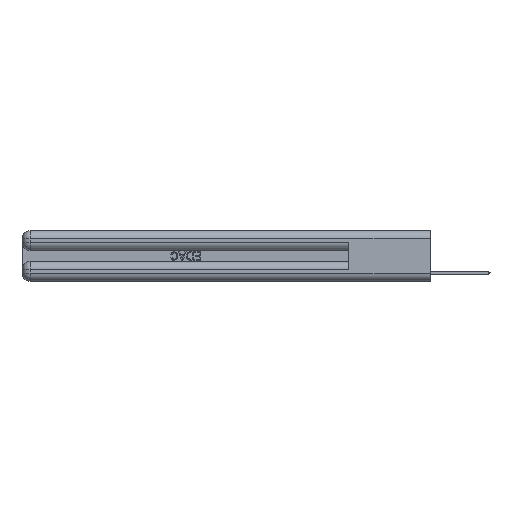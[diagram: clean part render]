
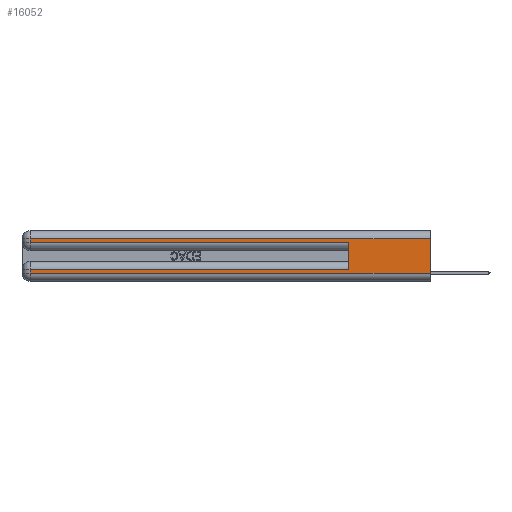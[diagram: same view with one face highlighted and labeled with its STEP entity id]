
A CAD part, left-side view. The second image highlights one B-rep face of the part: STEP entity #16052.
In plain terms, the highlighted planar face has unit normal (-1, 0, 0).
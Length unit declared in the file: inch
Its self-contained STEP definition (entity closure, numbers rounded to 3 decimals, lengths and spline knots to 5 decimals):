
#622 = VECTOR ( 'NONE', #1805, 39.37008 ) ;
#898 = VERTEX_POINT ( 'NONE', #18366 ) ;
#1225 = PLANE ( 'NONE',  #11989 ) ;
#1238 = DIRECTION ( 'NONE',  ( 0., 0., -1. ) ) ;
#1465 = DIRECTION ( 'NONE',  ( 0., 1., 0. ) ) ;
#1669 = CARTESIAN_POINT ( 'NONE',  ( 0., 2.94, 0.06 ) ) ;
#1805 = DIRECTION ( 'NONE',  ( 0., 0., -1. ) ) ;
#2607 = VECTOR ( 'NONE', #1238, 39.37008 ) ;
#2774 = CARTESIAN_POINT ( 'NONE',  ( 0., 0., 0.085 ) ) ;
#3349 = EDGE_CURVE ( 'NONE', #22937, #3726, #15953, .T. ) ;
#3726 = VERTEX_POINT ( 'NONE', #12110 ) ;
#3815 = ORIENTED_EDGE ( 'NONE', *, *, #12244, .T. ) ;
#4378 = EDGE_LOOP ( 'NONE', ( #17534, #11414, #22323, #23015, #10605, #10803, #24562, #3815 ) ) ;
#4987 = CARTESIAN_POINT ( 'NONE',  ( 0., 0., 0.285 ) ) ;
#5040 = DIRECTION ( 'NONE',  ( 0., 1., 0. ) ) ;
#6197 = CARTESIAN_POINT ( 'NONE',  ( 0., 0., 0.37 ) ) ;
#6233 = DIRECTION ( 'NONE',  ( 0., -1., 0. ) ) ;
#6467 = EDGE_CURVE ( 'NONE', #26370, #21898, #28335, .T. ) ;
#6953 = CARTESIAN_POINT ( 'NONE',  ( 0., 2.94, 0.085 ) ) ;
#8284 = CARTESIAN_POINT ( 'NONE',  ( 0., 0., 0.06 ) ) ;
#8873 = LINE ( 'NONE', #10384, #2607 ) ;
#9558 = EDGE_CURVE ( 'NONE', #898, #27114, #16126, .T. ) ;
#9632 = LINE ( 'NONE', #2774, #17637 ) ;
#9817 = DIRECTION ( 'NONE',  ( 0., -1., 0. ) ) ;
#10037 = VERTEX_POINT ( 'NONE', #25179 ) ;
#10089 = CARTESIAN_POINT ( 'NONE',  ( 0., 0., 0.37 ) ) ;
#10384 = CARTESIAN_POINT ( 'NONE',  ( 0., 2.94, 0.37 ) ) ;
#10605 = ORIENTED_EDGE ( 'NONE', *, *, #9558, .F. ) ;
#10803 = ORIENTED_EDGE ( 'NONE', *, *, #14807, .T. ) ;
#11414 = ORIENTED_EDGE ( 'NONE', *, *, #18991, .T. ) ;
#11421 = LINE ( 'NONE', #8284, #21848 ) ;
#11809 = LINE ( 'NONE', #4987, #20865 ) ;
#11989 = AXIS2_PLACEMENT_3D ( 'NONE', #10089, #21379, #21545 ) ;
#12110 = CARTESIAN_POINT ( 'NONE',  ( 0., 0., 0.06 ) ) ;
#12244 = EDGE_CURVE ( 'NONE', #21898, #3726, #11421, .T. ) ;
#13862 = CARTESIAN_POINT ( 'NONE',  ( 0., 0.6, 0.145 ) ) ;
#14266 = CARTESIAN_POINT ( 'NONE',  ( 0., 2.94, 0.31 ) ) ;
#14807 = EDGE_CURVE ( 'NONE', #898, #26370, #9632, .T. ) ;
#15558 = DIRECTION ( 'NONE',  ( 0., 0., -1. ) ) ;
#15953 = LINE ( 'NONE', #6197, #622 ) ;
#16052 = ADVANCED_FACE ( 'NONE', ( #24059 ), #1225, .F. ) ;
#16080 = DIRECTION ( 'NONE',  ( 0., 0., 1. ) ) ;
#16126 = LINE ( 'NONE', #13862, #21361 ) ;
#16150 = CARTESIAN_POINT ( 'NONE',  ( 0., 0.6, 0.285 ) ) ;
#17100 = EDGE_CURVE ( 'NONE', #10037, #27114, #11809, .T. ) ;
#17534 = ORIENTED_EDGE ( 'NONE', *, *, #3349, .F. ) ;
#17637 = VECTOR ( 'NONE', #5040, 39.37008 ) ;
#18366 = CARTESIAN_POINT ( 'NONE',  ( 0., 0.6, 0.085 ) ) ;
#18991 = EDGE_CURVE ( 'NONE', #22937, #21808, #20765, .T. ) ;
#20765 = LINE ( 'NONE', #28618, #27378 ) ;
#20865 = VECTOR ( 'NONE', #6233, 39.37008 ) ;
#21361 = VECTOR ( 'NONE', #16080, 39.37008 ) ;
#21379 = DIRECTION ( 'NONE',  ( 1., 0., 0. ) ) ;
#21545 = DIRECTION ( 'NONE',  ( 0., 0., -1. ) ) ;
#21808 = VERTEX_POINT ( 'NONE', #14266 ) ;
#21848 = VECTOR ( 'NONE', #9817, 39.37008 ) ;
#21898 = VERTEX_POINT ( 'NONE', #1669 ) ;
#22323 = ORIENTED_EDGE ( 'NONE', *, *, #22998, .T. ) ;
#22937 = VERTEX_POINT ( 'NONE', #28007 ) ;
#22998 = EDGE_CURVE ( 'NONE', #21808, #10037, #8873, .T. ) ;
#23015 = ORIENTED_EDGE ( 'NONE', *, *, #17100, .T. ) ;
#24059 = FACE_OUTER_BOUND ( 'NONE', #4378, .T. ) ;
#24310 = CARTESIAN_POINT ( 'NONE',  ( 0., 2.94, 0.37 ) ) ;
#24562 = ORIENTED_EDGE ( 'NONE', *, *, #6467, .T. ) ;
#25179 = CARTESIAN_POINT ( 'NONE',  ( 0., 2.94, 0.285 ) ) ;
#26370 = VERTEX_POINT ( 'NONE', #6953 ) ;
#27114 = VERTEX_POINT ( 'NONE', #16150 ) ;
#27378 = VECTOR ( 'NONE', #1465, 39.37008 ) ;
#28007 = CARTESIAN_POINT ( 'NONE',  ( 0., 0., 0.31 ) ) ;
#28335 = LINE ( 'NONE', #24310, #28707 ) ;
#28618 = CARTESIAN_POINT ( 'NONE',  ( 0., 0., 0.31 ) ) ;
#28707 = VECTOR ( 'NONE', #15558, 39.37008 ) ;
